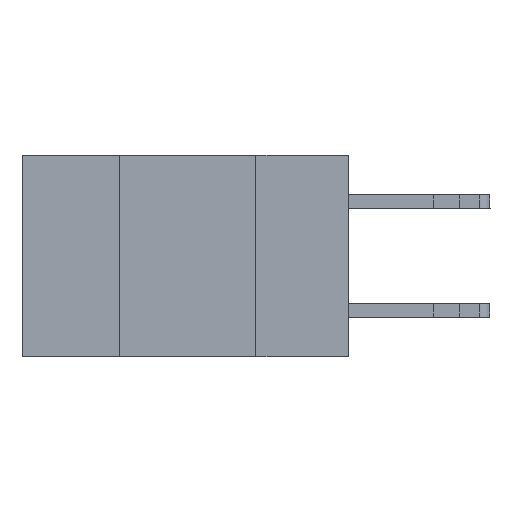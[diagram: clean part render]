
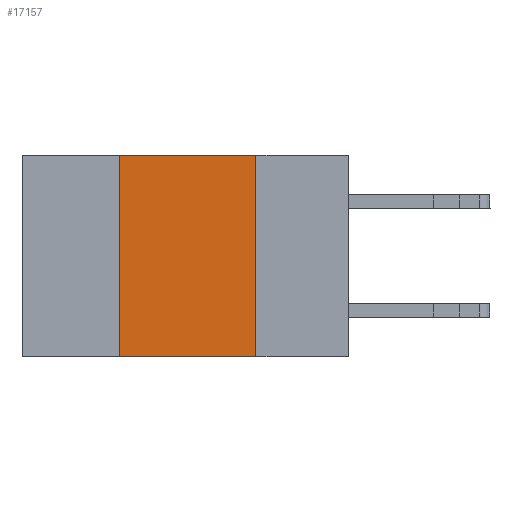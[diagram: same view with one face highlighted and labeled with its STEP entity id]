
A CAD part, left-side view. The second image highlights one B-rep face of the part: STEP entity #17157.
In plain terms, the highlighted planar face has unit normal (-1, 0, 0).
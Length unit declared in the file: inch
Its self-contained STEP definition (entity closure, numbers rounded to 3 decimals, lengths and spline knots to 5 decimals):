
#282 = FACE_OUTER_BOUND ( 'NONE', #10075, .T. ) ;
#365 = PLANE ( 'NONE',  #3996 ) ;
#541 = LINE ( 'NONE', #12737, #9802 ) ;
#2149 = VERTEX_POINT ( 'NONE', #8079 ) ;
#3371 = EDGE_CURVE ( 'NONE', #2149, #16862, #541, .T. ) ;
#3550 = ORIENTED_EDGE ( 'NONE', *, *, #10504, .F. ) ;
#3977 = EDGE_CURVE ( 'NONE', #16862, #17297, #17052, .T. ) ;
#3996 = AXIS2_PLACEMENT_3D ( 'NONE', #5350, #9402, #13357 ) ;
#4009 = LINE ( 'NONE', #11645, #9637 ) ;
#4812 = VERTEX_POINT ( 'NONE', #6362 ) ;
#5350 = CARTESIAN_POINT ( 'NONE',  ( 0., 0.6, 0. ) ) ;
#5853 = LINE ( 'NONE', #6286, #8245 ) ;
#6286 = CARTESIAN_POINT ( 'NONE',  ( 0., 0.6, -0.37 ) ) ;
#6362 = CARTESIAN_POINT ( 'NONE',  ( 0., 0.42, -0.37 ) ) ;
#8079 = CARTESIAN_POINT ( 'NONE',  ( 0., 0.42, 0. ) ) ;
#8245 = VECTOR ( 'NONE', #15434, 39.37008 ) ;
#8461 = VECTOR ( 'NONE', #14237, 39.37008 ) ;
#8695 = CARTESIAN_POINT ( 'NONE',  ( 0., 0.17, -0.37 ) ) ;
#8716 = CARTESIAN_POINT ( 'NONE',  ( 0., 0.17, 0. ) ) ;
#8981 = ORIENTED_EDGE ( 'NONE', *, *, #3977, .F. ) ;
#9050 = ORIENTED_EDGE ( 'NONE', *, *, #3371, .F. ) ;
#9402 = DIRECTION ( 'NONE',  ( 1., 0., 0. ) ) ;
#9637 = VECTOR ( 'NONE', #17011, 39.37008 ) ;
#9802 = VECTOR ( 'NONE', #11231, 39.37008 ) ;
#10075 = EDGE_LOOP ( 'NONE', ( #8981, #9050, #3550, #10363 ) ) ;
#10363 = ORIENTED_EDGE ( 'NONE', *, *, #11562, .T. ) ;
#10504 = EDGE_CURVE ( 'NONE', #4812, #2149, #4009, .T. ) ;
#11231 = DIRECTION ( 'NONE',  ( 0., -1., 0. ) ) ;
#11562 = EDGE_CURVE ( 'NONE', #4812, #17297, #5853, .T. ) ;
#11645 = CARTESIAN_POINT ( 'NONE',  ( 0., 0.42, -0.37 ) ) ;
#12737 = CARTESIAN_POINT ( 'NONE',  ( 0., 0.6, 0. ) ) ;
#13357 = DIRECTION ( 'NONE',  ( 0., 0., -1. ) ) ;
#14237 = DIRECTION ( 'NONE',  ( 0., 0., -1. ) ) ;
#15434 = DIRECTION ( 'NONE',  ( 0., -1., 0. ) ) ;
#16862 = VERTEX_POINT ( 'NONE', #8716 ) ;
#17011 = DIRECTION ( 'NONE',  ( 0., 0., 1. ) ) ;
#17052 = LINE ( 'NONE', #17138, #8461 ) ;
#17138 = CARTESIAN_POINT ( 'NONE',  ( 0., 0.17, -0.37 ) ) ;
#17157 = ADVANCED_FACE ( 'NONE', ( #282 ), #365, .F. ) ;
#17297 = VERTEX_POINT ( 'NONE', #8695 ) ;
